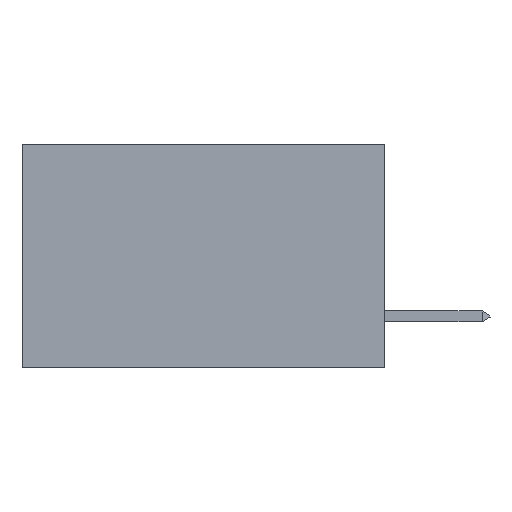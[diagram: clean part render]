
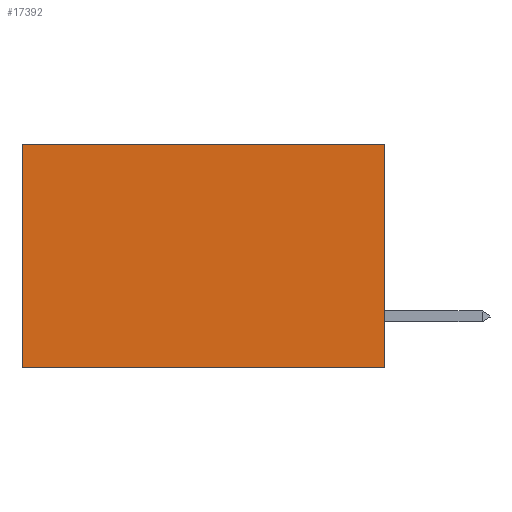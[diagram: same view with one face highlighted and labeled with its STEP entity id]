
A CAD part, left-side view. The second image highlights one B-rep face of the part: STEP entity #17392.
In plain terms, the highlighted planar face has unit normal (-1, 0, 0).
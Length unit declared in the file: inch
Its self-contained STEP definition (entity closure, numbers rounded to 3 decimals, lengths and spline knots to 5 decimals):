
#1809 = CARTESIAN_POINT ( 'NONE',  ( 0.2875, 0., 0. ) ) ;
#2117 = CARTESIAN_POINT ( 'NONE',  ( 0.2875, 0.6, 0. ) ) ;
#5734 = VECTOR ( 'NONE', #14015, 39.37008 ) ;
#6507 = VERTEX_POINT ( 'NONE', #2117 ) ;
#7493 = AXIS2_PLACEMENT_3D ( 'NONE', #34040, #23792, #12994 ) ;
#8832 = VERTEX_POINT ( 'NONE', #38512 ) ;
#10974 = VECTOR ( 'NONE', #30157, 39.37008 ) ;
#11506 = ORIENTED_EDGE ( 'NONE', *, *, #34180, .F. ) ;
#11654 = VECTOR ( 'NONE', #44612, 39.37008 ) ;
#12994 = DIRECTION ( 'NONE',  ( 0., 0., -1. ) ) ;
#14015 = DIRECTION ( 'NONE',  ( 0., 1., 0. ) ) ;
#14541 = EDGE_LOOP ( 'NONE', ( #30835, #18737, #11506, #15337 ) ) ;
#14627 = LINE ( 'NONE', #28696, #35648 ) ;
#15337 = ORIENTED_EDGE ( 'NONE', *, *, #31512, .T. ) ;
#17392 = ADVANCED_FACE ( 'NONE', ( #37538 ), #19455, .F. ) ;
#18703 = EDGE_CURVE ( 'NONE', #46535, #21429, #35265, .T. ) ;
#18737 = ORIENTED_EDGE ( 'NONE', *, *, #18703, .F. ) ;
#19455 = PLANE ( 'NONE',  #7493 ) ;
#21318 = LINE ( 'NONE', #1809, #10974 ) ;
#21409 = LINE ( 'NONE', #44949, #11654 ) ;
#21429 = VERTEX_POINT ( 'NONE', #27848 ) ;
#23792 = DIRECTION ( 'NONE',  ( 1., 0., 0. ) ) ;
#27848 = CARTESIAN_POINT ( 'NONE',  ( 0.2875, 0.6, -0.37 ) ) ;
#28696 = CARTESIAN_POINT ( 'NONE',  ( 0.2875, 0., 0. ) ) ;
#29197 = EDGE_CURVE ( 'NONE', #6507, #21429, #21409, .T. ) ;
#30157 = DIRECTION ( 'NONE',  ( 0., 0., -1. ) ) ;
#30835 = ORIENTED_EDGE ( 'NONE', *, *, #29197, .T. ) ;
#31512 = EDGE_CURVE ( 'NONE', #8832, #6507, #14627, .T. ) ;
#32763 = DIRECTION ( 'NONE',  ( 0., 1., 0. ) ) ;
#34040 = CARTESIAN_POINT ( 'NONE',  ( 0.2875, 0., 0. ) ) ;
#34180 = EDGE_CURVE ( 'NONE', #8832, #46535, #21318, .T. ) ;
#35265 = LINE ( 'NONE', #35551, #5734 ) ;
#35313 = CARTESIAN_POINT ( 'NONE',  ( 0.2875, 0., -0.37 ) ) ;
#35551 = CARTESIAN_POINT ( 'NONE',  ( 0.2875, 0., -0.37 ) ) ;
#35648 = VECTOR ( 'NONE', #32763, 39.37008 ) ;
#37538 = FACE_OUTER_BOUND ( 'NONE', #14541, .T. ) ;
#38512 = CARTESIAN_POINT ( 'NONE',  ( 0.2875, 0., 0. ) ) ;
#44612 = DIRECTION ( 'NONE',  ( 0., 0., -1. ) ) ;
#44949 = CARTESIAN_POINT ( 'NONE',  ( 0.2875, 0.6, 0. ) ) ;
#46535 = VERTEX_POINT ( 'NONE', #35313 ) ;
